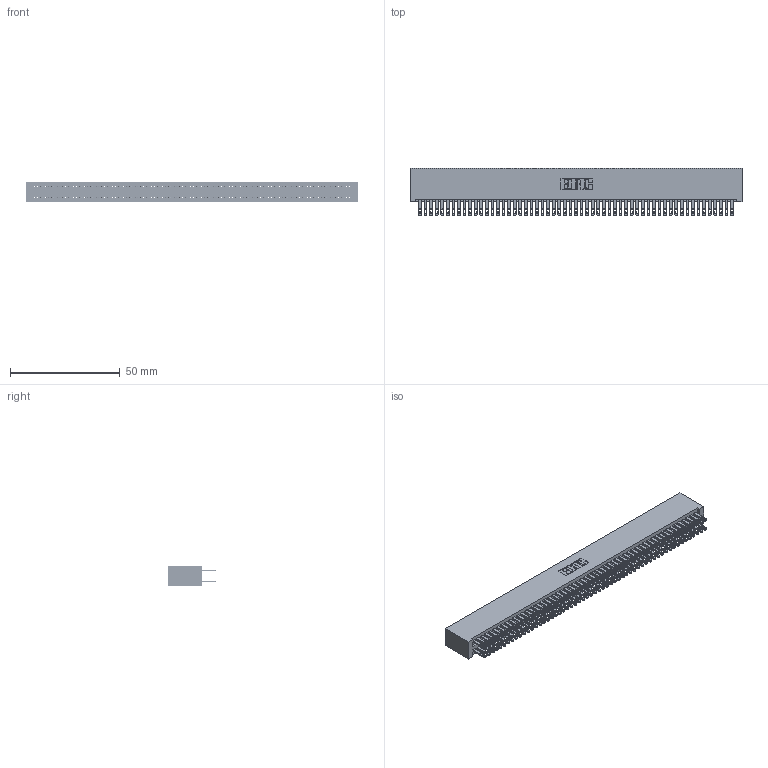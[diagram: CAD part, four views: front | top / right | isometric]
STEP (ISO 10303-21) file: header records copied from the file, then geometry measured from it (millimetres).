
FILE_DESCRIPTION (( 'STEP AP203' ), '1' );
FILE_NAME ('345-114-500-201.STEP', '2018-10-07T18:05:58', ( '' ), ( '' ), 'SwSTEP 2.0', 'SolidWorks 2016', '' );
FILE_SCHEMA (( 'CONFIG_CONTROL_DESIGN' ));
Length unit declared in the file: inch
Products named in the file (3): 345 Part_No Mounting Lugs; 345-114-500-201; 345-292-001_345-293-100
Assembly tree (115 placements, depth 2):
  345-114-500-201
    345 Part_No Mounting Lugs
    345-292-001_345-293-100  x114
Bounding box: 151.38 x 21.51 x 9.4 mm (x, y, z)
Volume: 15809.1 mm3; surface area: 25125 mm2
Topology: 115 solids, 115 shells, 5362 faces, 16391 edges, 10926 vertices
Faces by surface type: plane 3154, cylinder 2208
Entity records: 42357 total; most frequent: CARTESIAN_POINT 7084, ORIENTED_EDGE 7018, DIRECTION 6225, EDGE_CURVE 3509, VECTOR 3153, LINE 3153, VERTEX_POINT 2338, AXIS2_PLACEMENT_3D 1536
